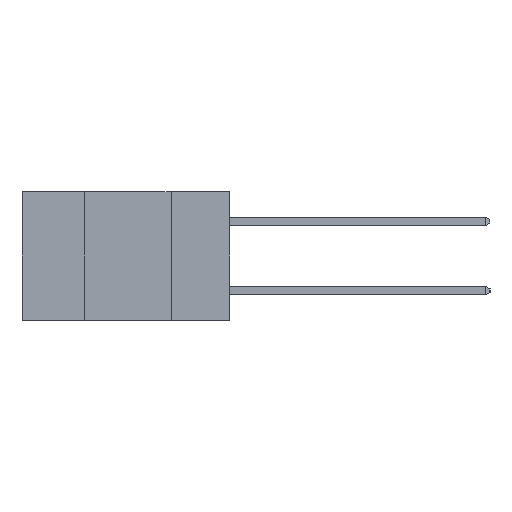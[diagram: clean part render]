
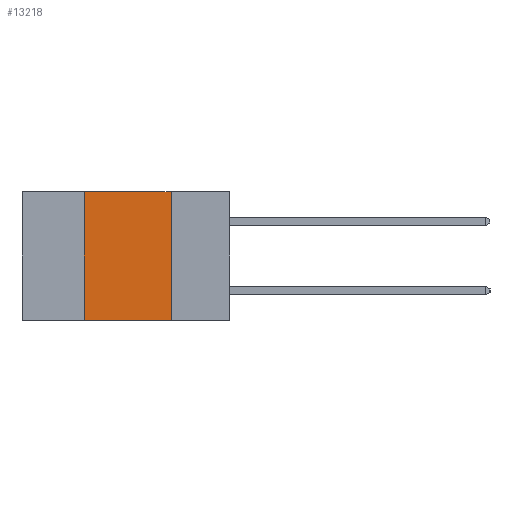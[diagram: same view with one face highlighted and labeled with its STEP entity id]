
A CAD part, left-side view. The second image highlights one B-rep face of the part: STEP entity #13218.
In plain terms, the highlighted planar face has unit normal (-1, 0, 0).
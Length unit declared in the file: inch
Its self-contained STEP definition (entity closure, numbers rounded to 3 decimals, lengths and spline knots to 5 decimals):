
#717 = CARTESIAN_POINT ( 'NONE',  ( 0., 0.42, 0. ) ) ;
#821 = CARTESIAN_POINT ( 'NONE',  ( 0., 0.17, -0.37 ) ) ;
#1317 = VECTOR ( 'NONE', #5366, 39.37008 ) ;
#1357 = EDGE_CURVE ( 'NONE', #10060, #8679, #7406, .T. ) ;
#1633 = VERTEX_POINT ( 'NONE', #8764 ) ;
#1838 = CARTESIAN_POINT ( 'NONE',  ( 0., 0.6, 0. ) ) ;
#1891 = VECTOR ( 'NONE', #11798, 39.37008 ) ;
#2195 = LINE ( 'NONE', #11769, #1891 ) ;
#2415 = ORIENTED_EDGE ( 'NONE', *, *, #1357, .F. ) ;
#2461 = CARTESIAN_POINT ( 'NONE',  ( 0., 0.6, -0.37 ) ) ;
#2914 = DIRECTION ( 'NONE',  ( 0., 0., -1. ) ) ;
#3608 = DIRECTION ( 'NONE',  ( 0., -1., 0. ) ) ;
#4543 = VECTOR ( 'NONE', #10970, 39.37008 ) ;
#5233 = FACE_OUTER_BOUND ( 'NONE', #7263, .T. ) ;
#5366 = DIRECTION ( 'NONE',  ( 0., -1., 0. ) ) ;
#5393 = CARTESIAN_POINT ( 'NONE',  ( 0., 0.6, 0. ) ) ;
#5456 = CARTESIAN_POINT ( 'NONE',  ( 0., 0.17, 0. ) ) ;
#7263 = EDGE_LOOP ( 'NONE', ( #2415, #10528, #13450, #11087 ) ) ;
#7406 = LINE ( 'NONE', #10960, #4543 ) ;
#8037 = EDGE_CURVE ( 'NONE', #1633, #12509, #2195, .T. ) ;
#8641 = AXIS2_PLACEMENT_3D ( 'NONE', #1838, #9217, #2914 ) ;
#8679 = VERTEX_POINT ( 'NONE', #821 ) ;
#8764 = CARTESIAN_POINT ( 'NONE',  ( 0., 0.42, -0.37 ) ) ;
#9060 = LINE ( 'NONE', #2461, #10845 ) ;
#9085 = LINE ( 'NONE', #5393, #1317 ) ;
#9217 = DIRECTION ( 'NONE',  ( 1., 0., 0. ) ) ;
#10060 = VERTEX_POINT ( 'NONE', #5456 ) ;
#10072 = EDGE_CURVE ( 'NONE', #12509, #10060, #9085, .T. ) ;
#10528 = ORIENTED_EDGE ( 'NONE', *, *, #10072, .F. ) ;
#10845 = VECTOR ( 'NONE', #3608, 39.37008 ) ;
#10960 = CARTESIAN_POINT ( 'NONE',  ( 0., 0.17, -0.37 ) ) ;
#10970 = DIRECTION ( 'NONE',  ( 0., 0., -1. ) ) ;
#11087 = ORIENTED_EDGE ( 'NONE', *, *, #11718, .T. ) ;
#11718 = EDGE_CURVE ( 'NONE', #1633, #8679, #9060, .T. ) ;
#11769 = CARTESIAN_POINT ( 'NONE',  ( 0., 0.42, -0.37 ) ) ;
#11798 = DIRECTION ( 'NONE',  ( 0., 0., 1. ) ) ;
#12509 = VERTEX_POINT ( 'NONE', #717 ) ;
#13218 = ADVANCED_FACE ( 'NONE', ( #5233 ), #13239, .F. ) ;
#13239 = PLANE ( 'NONE',  #8641 ) ;
#13450 = ORIENTED_EDGE ( 'NONE', *, *, #8037, .F. ) ;
